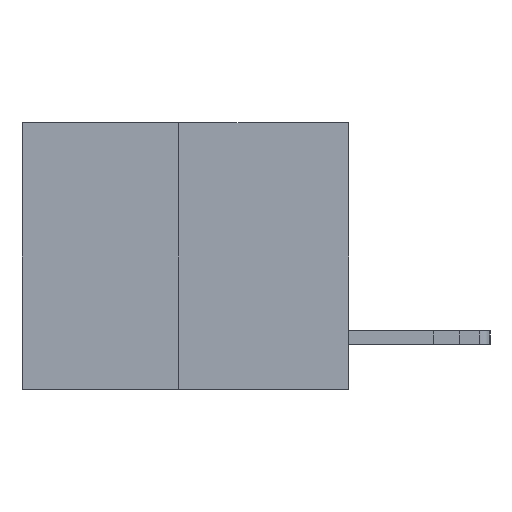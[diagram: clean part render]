
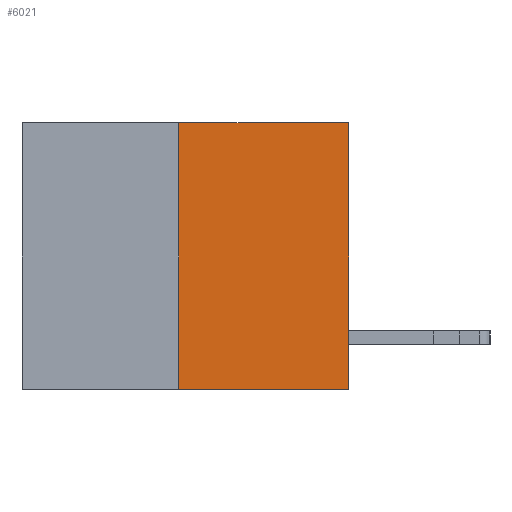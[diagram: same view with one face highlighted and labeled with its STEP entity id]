
A CAD part, left-side view. The second image highlights one B-rep face of the part: STEP entity #6021.
In plain terms, the highlighted planar face has unit normal (-1, 0, 0).
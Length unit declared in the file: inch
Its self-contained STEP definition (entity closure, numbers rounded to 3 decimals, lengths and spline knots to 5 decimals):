
#47 = DIRECTION ( 'NONE',  ( 0., 0., 1. ) ) ;
#81 = CARTESIAN_POINT ( 'NONE',  ( 0., 0., 0. ) ) ;
#121 = FACE_OUTER_BOUND ( 'NONE', #9359, .T. ) ;
#829 = DIRECTION ( 'NONE',  ( 0., -1., 0. ) ) ;
#1083 = ORIENTED_EDGE ( 'NONE', *, *, #14091, .T. ) ;
#1094 = CARTESIAN_POINT ( 'NONE',  ( 0., 0.312, -0.49 ) ) ;
#1561 = CARTESIAN_POINT ( 'NONE',  ( 0., 0., -0.49 ) ) ;
#2031 = AXIS2_PLACEMENT_3D ( 'NONE', #7330, #2997, #11886 ) ;
#2261 = VERTEX_POINT ( 'NONE', #1561 ) ;
#2721 = CARTESIAN_POINT ( 'NONE',  ( 0., 0.312, -0.49 ) ) ;
#2997 = DIRECTION ( 'NONE',  ( 1., 0., 0. ) ) ;
#3428 = LINE ( 'NONE', #7523, #14497 ) ;
#3883 = PLANE ( 'NONE',  #2031 ) ;
#4921 = EDGE_CURVE ( 'NONE', #11591, #2261, #6726, .T. ) ;
#5030 = EDGE_CURVE ( 'NONE', #5354, #13293, #12279, .T. ) ;
#5354 = VERTEX_POINT ( 'NONE', #9717 ) ;
#5443 = VECTOR ( 'NONE', #6916, 39.37008 ) ;
#6021 = ADVANCED_FACE ( 'NONE', ( #121 ), #3883, .F. ) ;
#6104 = EDGE_CURVE ( 'NONE', #11591, #5354, #10810, .T. ) ;
#6431 = ORIENTED_EDGE ( 'NONE', *, *, #4921, .T. ) ;
#6434 = ORIENTED_EDGE ( 'NONE', *, *, #6104, .F. ) ;
#6726 = LINE ( 'NONE', #12442, #11212 ) ;
#6916 = DIRECTION ( 'NONE',  ( 0., -1., 0. ) ) ;
#7330 = CARTESIAN_POINT ( 'NONE',  ( 0., 0.6, 0. ) ) ;
#7523 = CARTESIAN_POINT ( 'NONE',  ( 0., 0., 0. ) ) ;
#7917 = CARTESIAN_POINT ( 'NONE',  ( 0., 0.6, 0. ) ) ;
#9359 = EDGE_LOOP ( 'NONE', ( #6434, #6431, #1083, #9873 ) ) ;
#9717 = CARTESIAN_POINT ( 'NONE',  ( 0., 0.312, 0. ) ) ;
#9866 = DIRECTION ( 'NONE',  ( 0., 0., 1. ) ) ;
#9873 = ORIENTED_EDGE ( 'NONE', *, *, #5030, .F. ) ;
#10810 = LINE ( 'NONE', #1094, #10983 ) ;
#10983 = VECTOR ( 'NONE', #47, 39.37008 ) ;
#11212 = VECTOR ( 'NONE', #829, 39.37008 ) ;
#11591 = VERTEX_POINT ( 'NONE', #2721 ) ;
#11886 = DIRECTION ( 'NONE',  ( 0., 0., -1. ) ) ;
#12279 = LINE ( 'NONE', #7917, #5443 ) ;
#12442 = CARTESIAN_POINT ( 'NONE',  ( 0., 0.6, -0.49 ) ) ;
#13293 = VERTEX_POINT ( 'NONE', #81 ) ;
#14091 = EDGE_CURVE ( 'NONE', #2261, #13293, #3428, .T. ) ;
#14497 = VECTOR ( 'NONE', #9866, 39.37008 ) ;
